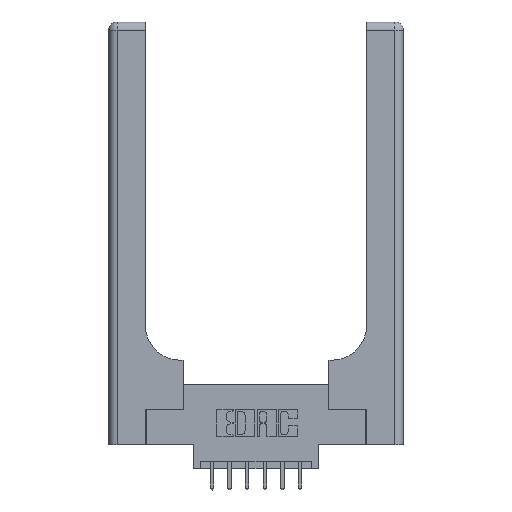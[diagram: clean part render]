
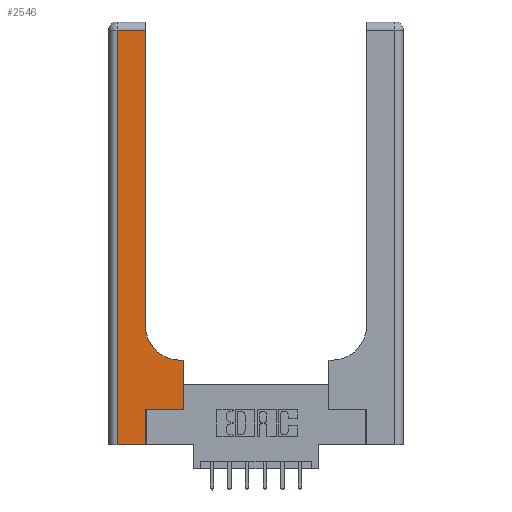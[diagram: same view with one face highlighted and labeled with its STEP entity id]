
A CAD part, top view. The second image highlights one B-rep face of the part: STEP entity #2546.
In plain terms, the highlighted planar face has unit normal (0, 0, 1).
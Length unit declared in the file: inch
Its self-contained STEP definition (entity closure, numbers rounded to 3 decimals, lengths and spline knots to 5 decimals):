
#179 = DIRECTION ( 'NONE',  ( 0., -1., 0. ) ) ;
#215 = LINE ( 'NONE', #1517, #11129 ) ;
#355 = EDGE_LOOP ( 'NONE', ( #11538, #8468, #12352, #4941, #4179, #4087, #6590, #5562, #4199 ) ) ;
#356 = LINE ( 'NONE', #13232, #8715 ) ;
#508 = CARTESIAN_POINT ( 'NONE',  ( 0.26, 0.6, 0.37 ) ) ;
#1083 = DIRECTION ( 'NONE',  ( -1., 0., 0. ) ) ;
#1517 = CARTESIAN_POINT ( 'NONE',  ( 0.265, 0.25, 0.37 ) ) ;
#2129 = VECTOR ( 'NONE', #9222, 39.37008 ) ;
#2435 = CARTESIAN_POINT ( 'NONE',  ( 0., 3., 0.37 ) ) ;
#2474 = LINE ( 'NONE', #508, #2129 ) ;
#2528 = PLANE ( 'NONE',  #4709 ) ;
#2546 = ADVANCED_FACE ( 'NONE', ( #12241 ), #2528, .F. ) ;
#2628 = VECTOR ( 'NONE', #1083, 39.37008 ) ;
#2803 = VERTEX_POINT ( 'NONE', #6226 ) ;
#2828 = CARTESIAN_POINT ( 'NONE',  ( 0.265, 0., 0.37 ) ) ;
#3140 = CARTESIAN_POINT ( 'NONE',  ( 0.26, 2.94, 0.37 ) ) ;
#3173 = CARTESIAN_POINT ( 'NONE',  ( 0.265, 0.25, 0.37 ) ) ;
#3577 = AXIS2_PLACEMENT_3D ( 'NONE', #6141, #13746, #7235 ) ;
#3629 = DIRECTION ( 'NONE',  ( -1., 0., 0. ) ) ;
#4087 = ORIENTED_EDGE ( 'NONE', *, *, #9590, .T. ) ;
#4169 = EDGE_CURVE ( 'NONE', #6182, #6695, #13964, .T. ) ;
#4179 = ORIENTED_EDGE ( 'NONE', *, *, #12197, .T. ) ;
#4199 = ORIENTED_EDGE ( 'NONE', *, *, #9249, .T. ) ;
#4349 = LINE ( 'NONE', #7471, #6902 ) ;
#4384 = DIRECTION ( 'NONE',  ( 1., 0., 0. ) ) ;
#4559 = CARTESIAN_POINT ( 'NONE',  ( 0.528, 0.25, 0.37 ) ) ;
#4641 = EDGE_CURVE ( 'NONE', #11311, #2803, #356, .T. ) ;
#4709 = AXIS2_PLACEMENT_3D ( 'NONE', #2435, #10155, #3629 ) ;
#4941 = ORIENTED_EDGE ( 'NONE', *, *, #5162, .T. ) ;
#5162 = EDGE_CURVE ( 'NONE', #2803, #13635, #10907, .T. ) ;
#5562 = ORIENTED_EDGE ( 'NONE', *, *, #8629, .T. ) ;
#6141 = CARTESIAN_POINT ( 'NONE',  ( 0.51, 0.85, 0.37 ) ) ;
#6182 = VERTEX_POINT ( 'NONE', #9389 ) ;
#6226 = CARTESIAN_POINT ( 'NONE',  ( 0.06, 0., 0.37 ) ) ;
#6470 = CARTESIAN_POINT ( 'NONE',  ( 0.528, 0.6, 0.37 ) ) ;
#6590 = ORIENTED_EDGE ( 'NONE', *, *, #12644, .T. ) ;
#6695 = VERTEX_POINT ( 'NONE', #3140 ) ;
#6902 = VECTOR ( 'NONE', #8572, 39.37008 ) ;
#7235 = DIRECTION ( 'NONE',  ( 1., 0., 0. ) ) ;
#7471 = CARTESIAN_POINT ( 'NONE',  ( 0.265, 0., 0.37 ) ) ;
#7749 = CARTESIAN_POINT ( 'NONE',  ( 0.06, 2.94, 0.37 ) ) ;
#8403 = LINE ( 'NONE', #10849, #2628 ) ;
#8468 = ORIENTED_EDGE ( 'NONE', *, *, #9376, .T. ) ;
#8572 = DIRECTION ( 'NONE',  ( 0., 1., 0. ) ) ;
#8629 = EDGE_CURVE ( 'NONE', #12827, #9932, #2474, .T. ) ;
#8705 = CARTESIAN_POINT ( 'NONE',  ( 0., 0., 0.37 ) ) ;
#8715 = VECTOR ( 'NONE', #179, 39.37008 ) ;
#8908 = VERTEX_POINT ( 'NONE', #3173 ) ;
#9057 = CARTESIAN_POINT ( 'NONE',  ( 0.26, 3., 0.37 ) ) ;
#9107 = DIRECTION ( 'NONE',  ( 0., 1., 0. ) ) ;
#9222 = DIRECTION ( 'NONE',  ( -1., 0., 0. ) ) ;
#9249 = EDGE_CURVE ( 'NONE', #9932, #6182, #9773, .T. ) ;
#9376 = EDGE_CURVE ( 'NONE', #6695, #11311, #8403, .T. ) ;
#9389 = CARTESIAN_POINT ( 'NONE',  ( 0.26, 0.85, 0.37 ) ) ;
#9590 = EDGE_CURVE ( 'NONE', #8908, #13506, #215, .T. ) ;
#9641 = CARTESIAN_POINT ( 'NONE',  ( 0.51, 0.6, 0.37 ) ) ;
#9773 = CIRCLE ( 'NONE', #3577, 0.25 ) ;
#9932 = VERTEX_POINT ( 'NONE', #9641 ) ;
#10121 = VECTOR ( 'NONE', #13646, 39.37008 ) ;
#10155 = DIRECTION ( 'NONE',  ( 0., 0., -1. ) ) ;
#10242 = DIRECTION ( 'NONE',  ( 1., 0., 0. ) ) ;
#10738 = VECTOR ( 'NONE', #9107, 39.37008 ) ;
#10849 = CARTESIAN_POINT ( 'NONE',  ( 0., 2.94, 0.37 ) ) ;
#10907 = LINE ( 'NONE', #8705, #13460 ) ;
#11129 = VECTOR ( 'NONE', #10242, 39.37008 ) ;
#11311 = VERTEX_POINT ( 'NONE', #7749 ) ;
#11538 = ORIENTED_EDGE ( 'NONE', *, *, #4169, .T. ) ;
#12197 = EDGE_CURVE ( 'NONE', #13635, #8908, #4349, .T. ) ;
#12241 = FACE_OUTER_BOUND ( 'NONE', #355, .T. ) ;
#12352 = ORIENTED_EDGE ( 'NONE', *, *, #4641, .T. ) ;
#12551 = CARTESIAN_POINT ( 'NONE',  ( 0.528, 0.25, 0.37 ) ) ;
#12644 = EDGE_CURVE ( 'NONE', #13506, #12827, #13680, .T. ) ;
#12827 = VERTEX_POINT ( 'NONE', #6470 ) ;
#13232 = CARTESIAN_POINT ( 'NONE',  ( 0.06, 3., 0.37 ) ) ;
#13460 = VECTOR ( 'NONE', #4384, 39.37008 ) ;
#13506 = VERTEX_POINT ( 'NONE', #4559 ) ;
#13635 = VERTEX_POINT ( 'NONE', #2828 ) ;
#13646 = DIRECTION ( 'NONE',  ( 0., 1., 0. ) ) ;
#13680 = LINE ( 'NONE', #12551, #10121 ) ;
#13746 = DIRECTION ( 'NONE',  ( 0., 0., -1. ) ) ;
#13964 = LINE ( 'NONE', #9057, #10738 ) ;
